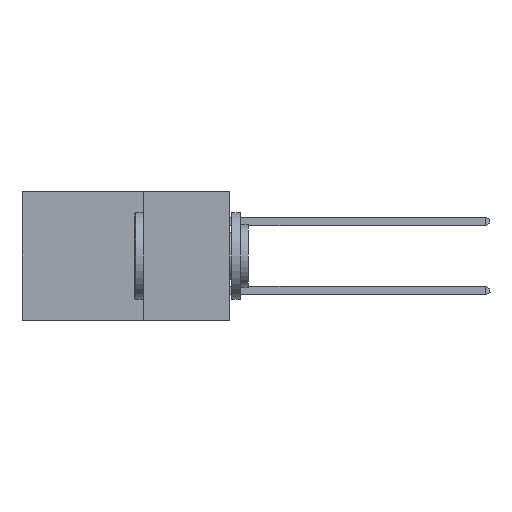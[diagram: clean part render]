
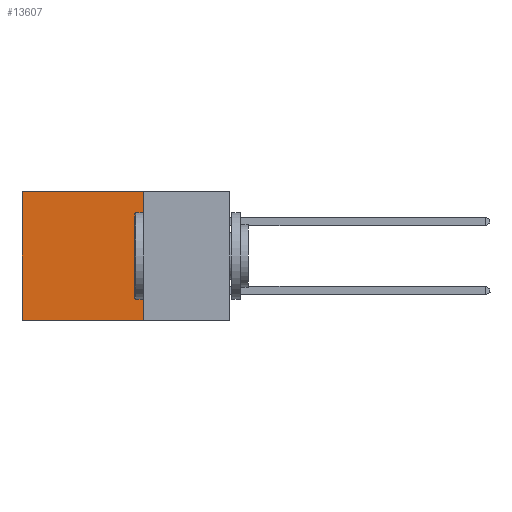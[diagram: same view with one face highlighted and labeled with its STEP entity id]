
A CAD part, left-side view. The second image highlights one B-rep face of the part: STEP entity #13607.
In plain terms, the highlighted planar face has unit normal (-1, 0, 0).
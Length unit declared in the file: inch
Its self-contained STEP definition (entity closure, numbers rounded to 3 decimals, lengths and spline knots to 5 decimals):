
#575 = FACE_OUTER_BOUND ( 'NONE', #18861, .T. ) ;
#2908 = DIRECTION ( 'NONE',  ( 1., 0., 0. ) ) ;
#3112 = CARTESIAN_POINT ( 'NONE',  ( 0.298, 0.6, 0. ) ) ;
#3226 = EDGE_CURVE ( 'NONE', #13490, #19134, #27089, .T. ) ;
#3401 = LINE ( 'NONE', #8511, #21395 ) ;
#5569 = LINE ( 'NONE', #18497, #17704 ) ;
#7331 = CARTESIAN_POINT ( 'NONE',  ( 0.298, 0.25, 0. ) ) ;
#7358 = AXIS2_PLACEMENT_3D ( 'NONE', #9666, #2908, #25997 ) ;
#8320 = DIRECTION ( 'NONE',  ( 0., 1., 0. ) ) ;
#8511 = CARTESIAN_POINT ( 'NONE',  ( 0.298, 0.25, -0.37 ) ) ;
#9639 = EDGE_CURVE ( 'NONE', #19134, #28136, #3401, .T. ) ;
#9666 = CARTESIAN_POINT ( 'NONE',  ( 0.298, 0.25, 0. ) ) ;
#11557 = LINE ( 'NONE', #17603, #24801 ) ;
#13184 = ORIENTED_EDGE ( 'NONE', *, *, #9639, .F. ) ;
#13401 = CARTESIAN_POINT ( 'NONE',  ( 0.298, 0.25, -0.37 ) ) ;
#13490 = VERTEX_POINT ( 'NONE', #7331 ) ;
#13607 = ADVANCED_FACE ( 'NONE', ( #575 ), #28693, .F. ) ;
#15284 = ORIENTED_EDGE ( 'NONE', *, *, #25037, .T. ) ;
#17603 = CARTESIAN_POINT ( 'NONE',  ( 0.298, 0.6, 0. ) ) ;
#17704 = VECTOR ( 'NONE', #21056, 39.37008 ) ;
#18497 = CARTESIAN_POINT ( 'NONE',  ( 0.298, 0.25, 0. ) ) ;
#18861 = EDGE_LOOP ( 'NONE', ( #15284, #13184, #19819, #27555 ) ) ;
#19134 = VERTEX_POINT ( 'NONE', #13401 ) ;
#19421 = VERTEX_POINT ( 'NONE', #3112 ) ;
#19819 = ORIENTED_EDGE ( 'NONE', *, *, #3226, .F. ) ;
#21056 = DIRECTION ( 'NONE',  ( 0., 1., 0. ) ) ;
#21058 = CARTESIAN_POINT ( 'NONE',  ( 0.298, 0.25, 0. ) ) ;
#21395 = VECTOR ( 'NONE', #8320, 39.37008 ) ;
#21861 = EDGE_CURVE ( 'NONE', #13490, #19421, #5569, .T. ) ;
#23408 = VECTOR ( 'NONE', #28118, 39.37008 ) ;
#24462 = DIRECTION ( 'NONE',  ( 0., 0., -1. ) ) ;
#24801 = VECTOR ( 'NONE', #24462, 39.37008 ) ;
#25037 = EDGE_CURVE ( 'NONE', #19421, #28136, #11557, .T. ) ;
#25997 = DIRECTION ( 'NONE',  ( 0., 0., -1. ) ) ;
#26506 = CARTESIAN_POINT ( 'NONE',  ( 0.298, 0.6, -0.37 ) ) ;
#27089 = LINE ( 'NONE', #21058, #23408 ) ;
#27555 = ORIENTED_EDGE ( 'NONE', *, *, #21861, .T. ) ;
#28118 = DIRECTION ( 'NONE',  ( 0., 0., -1. ) ) ;
#28136 = VERTEX_POINT ( 'NONE', #26506 ) ;
#28693 = PLANE ( 'NONE',  #7358 ) ;
